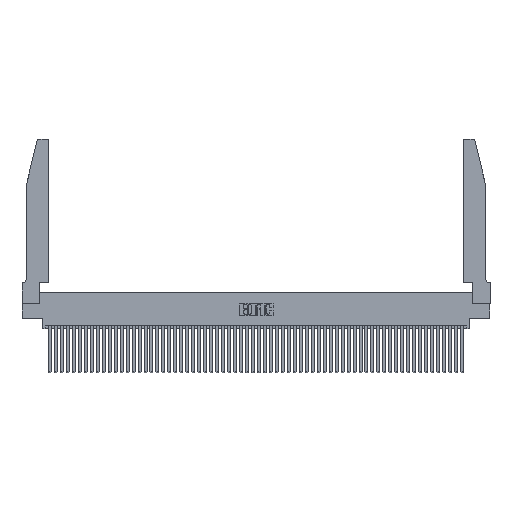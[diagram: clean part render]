
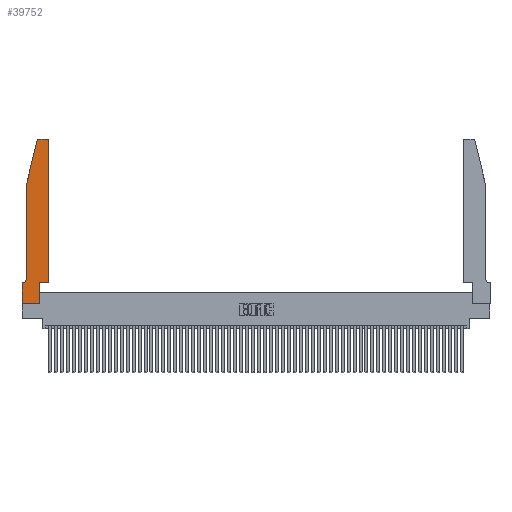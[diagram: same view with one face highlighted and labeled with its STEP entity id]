
A CAD part, top view. The second image highlights one B-rep face of the part: STEP entity #39752.
In plain terms, the highlighted planar face has unit normal (0, 0, 1).
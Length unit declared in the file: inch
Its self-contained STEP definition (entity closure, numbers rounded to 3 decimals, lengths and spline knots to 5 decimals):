
#1282 = VECTOR ( 'NONE', #6810, 39.37008 ) ;
#1326 = AXIS2_PLACEMENT_3D ( 'NONE', #51649, #25757, #19493 ) ;
#1918 = VECTOR ( 'NONE', #37824, 39.37008 ) ;
#2145 = CARTESIAN_POINT ( 'NONE',  ( 0.2865, 0.35, 0.37 ) ) ;
#2541 = VECTOR ( 'NONE', #50602, 39.37008 ) ;
#3259 = LINE ( 'NONE', #46321, #1918 ) ;
#3319 = DIRECTION ( 'NONE',  ( 0., 1., 0. ) ) ;
#3427 = CIRCLE ( 'NONE', #40583, 0.03 ) ;
#4482 = ORIENTED_EDGE ( 'NONE', *, *, #9212, .T. ) ;
#5652 = CIRCLE ( 'NONE', #34293, 0.03 ) ;
#6329 = EDGE_CURVE ( 'NONE', #9101, #31267, #37077, .T. ) ;
#6509 = ORIENTED_EDGE ( 'NONE', *, *, #27515, .T. ) ;
#6635 = LINE ( 'NONE', #29150, #28227 ) ;
#6810 = DIRECTION ( 'NONE',  ( 0., -1., 0. ) ) ;
#6944 = DIRECTION ( 'NONE',  ( 0., 0., 1. ) ) ;
#7048 = VECTOR ( 'NONE', #8993, 39.37008 ) ;
#7947 = LINE ( 'NONE', #12211, #52544 ) ;
#8814 = CARTESIAN_POINT ( 'NONE',  ( 0., 0., 0.37 ) ) ;
#8993 = DIRECTION ( 'NONE',  ( -1., 0., 0. ) ) ;
#9101 = VERTEX_POINT ( 'NONE', #14627 ) ;
#9212 = EDGE_CURVE ( 'NONE', #34645, #13690, #5652, .T. ) ;
#10033 = CIRCLE ( 'NONE', #1326, 0.07 ) ;
#10298 = VERTEX_POINT ( 'NONE', #22664 ) ;
#10828 = PLANE ( 'NONE',  #23835 ) ;
#11722 = CARTESIAN_POINT ( 'NONE',  ( 0.0755, 2., 0.37 ) ) ;
#11740 = VECTOR ( 'NONE', #31771, 39.37008 ) ;
#12192 = VERTEX_POINT ( 'NONE', #40082 ) ;
#12211 = CARTESIAN_POINT ( 'NONE',  ( 0., 0., 0.37 ) ) ;
#12242 = DIRECTION ( 'NONE',  ( 0., 1., 0. ) ) ;
#13565 = EDGE_CURVE ( 'NONE', #30219, #26213, #3259, .T. ) ;
#13690 = VERTEX_POINT ( 'NONE', #51573 ) ;
#14627 = CARTESIAN_POINT ( 'NONE',  ( 0., 0.35, 0.37 ) ) ;
#15313 = DIRECTION ( 'NONE',  ( 1., 0., 0. ) ) ;
#15354 = DIRECTION ( 'NONE',  ( 0., 0., 1. ) ) ;
#15834 = ORIENTED_EDGE ( 'NONE', *, *, #17508, .T. ) ;
#15871 = EDGE_CURVE ( 'NONE', #29105, #12192, #48948, .T. ) ;
#16707 = CARTESIAN_POINT ( 'NONE',  ( 0.0755, 2., 0.37 ) ) ;
#17234 = ORIENTED_EDGE ( 'NONE', *, *, #32249, .T. ) ;
#17508 = EDGE_CURVE ( 'NONE', #23376, #9101, #44196, .T. ) ;
#19452 = CARTESIAN_POINT ( 'NONE',  ( 0., 0.35, 0.37 ) ) ;
#19493 = DIRECTION ( 'NONE',  ( -1., 0., 0. ) ) ;
#19836 = ORIENTED_EDGE ( 'NONE', *, *, #15871, .T. ) ;
#22487 = EDGE_CURVE ( 'NONE', #28263, #29105, #34260, .T. ) ;
#22643 = CARTESIAN_POINT ( 'NONE',  ( 0.2605, 2.75, 0.37 ) ) ;
#22664 = CARTESIAN_POINT ( 'NONE',  ( 0.2865, 0., 0.37 ) ) ;
#23020 = CARTESIAN_POINT ( 'NONE',  ( 0.0755, 2., 0.37 ) ) ;
#23123 = CARTESIAN_POINT ( 'NONE',  ( 0.0055, 0.35, 0.37 ) ) ;
#23376 = VERTEX_POINT ( 'NONE', #23123 ) ;
#23835 = AXIS2_PLACEMENT_3D ( 'NONE', #19452, #41219, #15313 ) ;
#25757 = DIRECTION ( 'NONE',  ( 0., 0., -1. ) ) ;
#26041 = LINE ( 'NONE', #22643, #47694 ) ;
#26213 = VERTEX_POINT ( 'NONE', #29471 ) ;
#26992 = DIRECTION ( 'NONE',  ( -1., 0., 0. ) ) ;
#27127 = ORIENTED_EDGE ( 'NONE', *, *, #29547, .T. ) ;
#27236 = ORIENTED_EDGE ( 'NONE', *, *, #22487, .T. ) ;
#27515 = EDGE_CURVE ( 'NONE', #26213, #34645, #6635, .T. ) ;
#28227 = VECTOR ( 'NONE', #3319, 39.37008 ) ;
#28263 = VERTEX_POINT ( 'NONE', #42319 ) ;
#29105 = VERTEX_POINT ( 'NONE', #16707 ) ;
#29150 = CARTESIAN_POINT ( 'NONE',  ( 0.4505, 0.35, 0.37 ) ) ;
#29398 = ORIENTED_EDGE ( 'NONE', *, *, #6329, .T. ) ;
#29471 = CARTESIAN_POINT ( 'NONE',  ( 0.4505, 0.35, 0.37 ) ) ;
#29547 = EDGE_CURVE ( 'NONE', #39955, #28263, #3427, .T. ) ;
#30219 = VERTEX_POINT ( 'NONE', #2145 ) ;
#31062 = EDGE_CURVE ( 'NONE', #31267, #10298, #7947, .T. ) ;
#31267 = VERTEX_POINT ( 'NONE', #8814 ) ;
#31771 = DIRECTION ( 'NONE',  ( 0., -1., 0. ) ) ;
#32249 = EDGE_CURVE ( 'NONE', #13690, #39955, #26041, .T. ) ;
#32830 = CARTESIAN_POINT ( 'NONE',  ( 0.4205, 2.72, 0.37 ) ) ;
#32865 = FACE_OUTER_BOUND ( 'NONE', #40030, .T. ) ;
#33664 = CARTESIAN_POINT ( 'NONE',  ( 0.284, 2.75, 0.37 ) ) ;
#34260 = LINE ( 'NONE', #11722, #2541 ) ;
#34293 = AXIS2_PLACEMENT_3D ( 'NONE', #32830, #6944, #37160 ) ;
#34645 = VERTEX_POINT ( 'NONE', #36162 ) ;
#36162 = CARTESIAN_POINT ( 'NONE',  ( 0.4505, 2.72, 0.37 ) ) ;
#37077 = LINE ( 'NONE', #41354, #1282 ) ;
#37160 = DIRECTION ( 'NONE',  ( 1., 0., 0. ) ) ;
#37824 = DIRECTION ( 'NONE',  ( 1., 0., 0. ) ) ;
#39216 = CARTESIAN_POINT ( 'NONE',  ( 0.0755, 0.35, 0.37 ) ) ;
#39752 = ADVANCED_FACE ( 'NONE', ( #32865 ), #10828, .T. ) ;
#39955 = VERTEX_POINT ( 'NONE', #33664 ) ;
#40030 = EDGE_LOOP ( 'NONE', ( #17234, #27127, #27236, #19836, #40857, #15834, #29398, #42265, #47677, #51728, #6509, #4482 ) ) ;
#40082 = CARTESIAN_POINT ( 'NONE',  ( 0.0755, 0.42, 0.37 ) ) ;
#40583 = AXIS2_PLACEMENT_3D ( 'NONE', #41266, #15354, #45626 ) ;
#40857 = ORIENTED_EDGE ( 'NONE', *, *, #46388, .T. ) ;
#41219 = DIRECTION ( 'NONE',  ( 0., 0., 1. ) ) ;
#41266 = CARTESIAN_POINT ( 'NONE',  ( 0.284, 2.72, 0.37 ) ) ;
#41354 = CARTESIAN_POINT ( 'NONE',  ( 0., 0., 0.37 ) ) ;
#42265 = ORIENTED_EDGE ( 'NONE', *, *, #31062, .T. ) ;
#42302 = CARTESIAN_POINT ( 'NONE',  ( 0.2865, 0.35, 0.37 ) ) ;
#42319 = CARTESIAN_POINT ( 'NONE',  ( 0.25487, 2.72718, 0.37 ) ) ;
#42444 = DIRECTION ( 'NONE',  ( 1., 0., 0. ) ) ;
#42500 = LINE ( 'NONE', #42302, #52611 ) ;
#44196 = LINE ( 'NONE', #39216, #7048 ) ;
#45626 = DIRECTION ( 'NONE',  ( 1., 0., 0. ) ) ;
#46321 = CARTESIAN_POINT ( 'NONE',  ( 0.4505, 0.35, 0.37 ) ) ;
#46388 = EDGE_CURVE ( 'NONE', #12192, #23376, #10033, .T. ) ;
#47677 = ORIENTED_EDGE ( 'NONE', *, *, #50180, .T. ) ;
#47694 = VECTOR ( 'NONE', #26992, 39.37008 ) ;
#48948 = LINE ( 'NONE', #23020, #11740 ) ;
#50180 = EDGE_CURVE ( 'NONE', #10298, #30219, #42500, .T. ) ;
#50602 = DIRECTION ( 'NONE',  ( -0.239, -0.971, 0. ) ) ;
#51573 = CARTESIAN_POINT ( 'NONE',  ( 0.4205, 2.75, 0.37 ) ) ;
#51649 = CARTESIAN_POINT ( 'NONE',  ( 0.0055, 0.42, 0.37 ) ) ;
#51728 = ORIENTED_EDGE ( 'NONE', *, *, #13565, .T. ) ;
#52544 = VECTOR ( 'NONE', #42444, 39.37008 ) ;
#52611 = VECTOR ( 'NONE', #12242, 39.37008 ) ;
